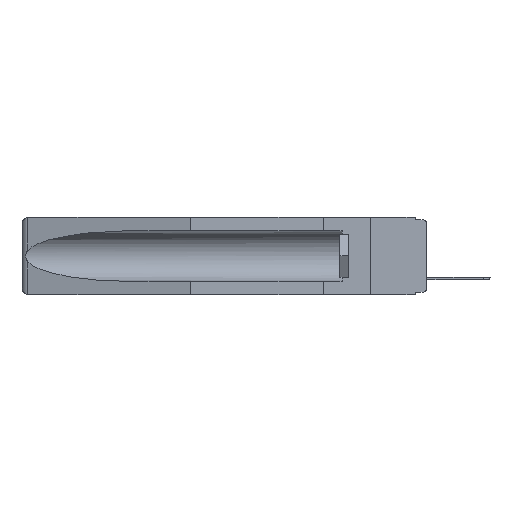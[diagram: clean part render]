
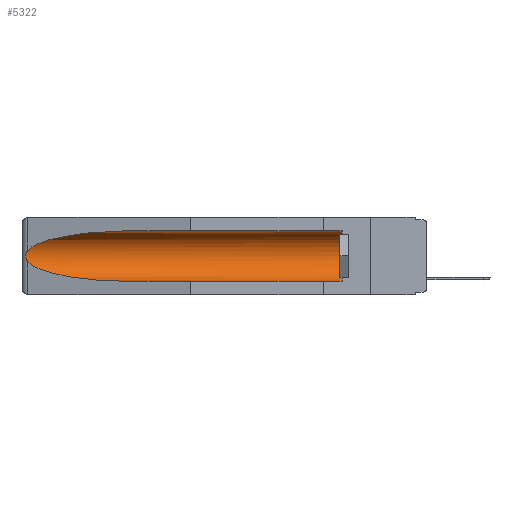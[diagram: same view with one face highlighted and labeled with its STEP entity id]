
A CAD part, left-side view. The second image highlights one B-rep face of the part: STEP entity #5322.
In plain terms, the highlighted cylindrical face has radius 2.857 mm (diameter 5.715 mm), a partial arc.
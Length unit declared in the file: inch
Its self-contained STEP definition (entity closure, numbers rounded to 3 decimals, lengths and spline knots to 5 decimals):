
#683 = CARTESIAN_POINT ( 'NONE',  ( 0.155, -0.30754, -0.284 ) ) ;
#787 = CARTESIAN_POINT ( 'NONE',  ( 0.26654, 1.53092, -0.15636 ) ) ;
#1100 = VECTOR ( 'NONE', #6120, 39.37008 ) ;
#1124 = ORIENTED_EDGE ( 'NONE', *, *, #7718, .T. ) ;
#1203 = CARTESIAN_POINT ( 'NONE',  ( 0.155, 0.126, -0.284 ) ) ;
#1211 = AXIS2_PLACEMENT_3D ( 'NONE', #17371, #18556, #12103 ) ;
#1513 = CARTESIAN_POINT ( 'NONE',  ( 0.155, 0.126, -0.059 ) ) ;
#2006 = CARTESIAN_POINT ( 'NONE',  ( 0.26537, 1.52718, -0.14972 ) ) ;
#2547 =( BOUNDED_CURVE ( )  B_SPLINE_CURVE ( 3, ( #9009, #9248, #4059, #2006 ),
 .UNSPECIFIED., .F., .F. ) 
 B_SPLINE_CURVE_WITH_KNOTS ( ( 4, 4 ),
 ( 4.71239, 6.08839 ),
 .UNSPECIFIED. ) 
 CURVE ( )  GEOMETRIC_REPRESENTATION_ITEM ( )  RATIONAL_B_SPLINE_CURVE ( ( 1., 0.848, 0.848, 1. ) ) 
 REPRESENTATION_ITEM ( '' )  );
#2720 = CARTESIAN_POINT ( 'NONE',  ( 0.26537, 1.52718, -0.19328 ) ) ;
#3109 = VERTEX_POINT ( 'NONE', #6705 ) ;
#3732 = FACE_OUTER_BOUND ( 'NONE', #19713, .T. ) ;
#4059 = CARTESIAN_POINT ( 'NONE',  ( 0.25451, 1.48313, -0.09465 ) ) ;
#4170 = VERTEX_POINT ( 'NONE', #1513 ) ;
#4382 = CARTESIAN_POINT ( 'NONE',  ( 0.2673, 1.5327, -0.16383 ) ) ;
#5322 = ADVANCED_FACE ( 'NONE', ( #3732 ), #6199, .F. ) ;
#6120 = DIRECTION ( 'NONE',  ( 0., 1., 0. ) ) ;
#6199 = CYLINDRICAL_SURFACE ( 'NONE', #1211, 0.1125 ) ;
#6209 = CARTESIAN_POINT ( 'NONE',  ( 0.26537, 1.52718, -0.19328 ) ) ;
#6258 = VECTOR ( 'NONE', #18378, 39.37008 ) ;
#6579 = ORIENTED_EDGE ( 'NONE', *, *, #21604, .T. ) ;
#6705 = CARTESIAN_POINT ( 'NONE',  ( 0.26537, 1.52718, -0.19328 ) ) ;
#6730 = B_SPLINE_CURVE_WITH_KNOTS ( 'NONE', 3,
 ( #16693, #16764, #787, #4382, #9739, #22152, #20535, #13294, #13214, #6209 ),
 .UNSPECIFIED., .F., .F.,
 ( 4, 2, 2, 2, 4 ),
 ( 0., 0.00029, 0.00058, 0.00087, 0.00117 ),
 .UNSPECIFIED. ) ;
#6990 = ORIENTED_EDGE ( 'NONE', *, *, #12426, .T. ) ;
#7102 = ORIENTED_EDGE ( 'NONE', *, *, #22781, .T. ) ;
#7718 = EDGE_CURVE ( 'NONE', #3109, #15463, #8443, .T. ) ;
#8443 =( BOUNDED_CURVE ( )  B_SPLINE_CURVE ( 3, ( #2720, #9881, #20753, #17055 ),
 .UNSPECIFIED., .F., .F. ) 
 B_SPLINE_CURVE_WITH_KNOTS ( ( 4, 4 ),
 ( 0.1948, 1.5708 ),
 .UNSPECIFIED. ) 
 CURVE ( )  GEOMETRIC_REPRESENTATION_ITEM ( )  RATIONAL_B_SPLINE_CURVE ( ( 1., 0.848, 0.848, 1. ) ) 
 REPRESENTATION_ITEM ( '' )  );
#8873 = LINE ( 'NONE', #683, #1100 ) ;
#8875 = CARTESIAN_POINT ( 'NONE',  ( 0.155, 1.07973, -0.059 ) ) ;
#9009 = CARTESIAN_POINT ( 'NONE',  ( 0.155, 1.07973, -0.059 ) ) ;
#9248 = CARTESIAN_POINT ( 'NONE',  ( 0.21114, 1.30732, -0.059 ) ) ;
#9261 = VERTEX_POINT ( 'NONE', #11685 ) ;
#9739 = CARTESIAN_POINT ( 'NONE',  ( 0.2675, 1.53308, -0.16763 ) ) ;
#9881 = CARTESIAN_POINT ( 'NONE',  ( 0.25451, 1.48313, -0.24835 ) ) ;
#10715 = LINE ( 'NONE', #11096, #6258 ) ;
#10975 = DIRECTION ( 'NONE',  ( 0., -1., 0. ) ) ;
#11096 = CARTESIAN_POINT ( 'NONE',  ( 0.155, -0.30754, -0.059 ) ) ;
#11420 = ORIENTED_EDGE ( 'NONE', *, *, #17907, .T. ) ;
#11685 = CARTESIAN_POINT ( 'NONE',  ( 0.26537, 1.52718, -0.14972 ) ) ;
#12015 = ORIENTED_EDGE ( 'NONE', *, *, #21710, .F. ) ;
#12040 = CARTESIAN_POINT ( 'NONE',  ( 0.155, 1.07973, -0.284 ) ) ;
#12103 = DIRECTION ( 'NONE',  ( 0., 0., 1. ) ) ;
#12426 = EDGE_CURVE ( 'NONE', #9261, #3109, #6730, .T. ) ;
#12588 = AXIS2_PLACEMENT_3D ( 'NONE', #14157, #10975, #19679 ) ;
#13214 = CARTESIAN_POINT ( 'NONE',  ( 0.26597, 1.5296, -0.19026 ) ) ;
#13294 = CARTESIAN_POINT ( 'NONE',  ( 0.26655, 1.53094, -0.18657 ) ) ;
#13748 = VERTEX_POINT ( 'NONE', #1203 ) ;
#14157 = CARTESIAN_POINT ( 'NONE',  ( 0.155, 0.126, -0.1715 ) ) ;
#15463 = VERTEX_POINT ( 'NONE', #12040 ) ;
#16693 = CARTESIAN_POINT ( 'NONE',  ( 0.26537, 1.52718, -0.14972 ) ) ;
#16764 = CARTESIAN_POINT ( 'NONE',  ( 0.26597, 1.52961, -0.15275 ) ) ;
#17055 = CARTESIAN_POINT ( 'NONE',  ( 0.155, 1.07973, -0.284 ) ) ;
#17371 = CARTESIAN_POINT ( 'NONE',  ( 0.155, -0.30754, -0.1715 ) ) ;
#17907 = EDGE_CURVE ( 'NONE', #4170, #18477, #10715, .T. ) ;
#18153 = CIRCLE ( 'NONE', #12588, 0.1125 ) ;
#18378 = DIRECTION ( 'NONE',  ( 0., 1., 0. ) ) ;
#18477 = VERTEX_POINT ( 'NONE', #8875 ) ;
#18556 = DIRECTION ( 'NONE',  ( 0., 1., 0. ) ) ;
#19679 = DIRECTION ( 'NONE',  ( 0., 0., 1. ) ) ;
#19713 = EDGE_LOOP ( 'NONE', ( #6579, #6990, #1124, #12015, #7102, #11420 ) ) ;
#20535 = CARTESIAN_POINT ( 'NONE',  ( 0.2673, 1.53269, -0.17917 ) ) ;
#20753 = CARTESIAN_POINT ( 'NONE',  ( 0.21114, 1.30732, -0.284 ) ) ;
#21604 = EDGE_CURVE ( 'NONE', #18477, #9261, #2547, .T. ) ;
#21710 = EDGE_CURVE ( 'NONE', #13748, #15463, #8873, .T. ) ;
#22152 = CARTESIAN_POINT ( 'NONE',  ( 0.2675, 1.53308, -0.17534 ) ) ;
#22781 = EDGE_CURVE ( 'NONE', #13748, #4170, #18153, .T. ) ;
